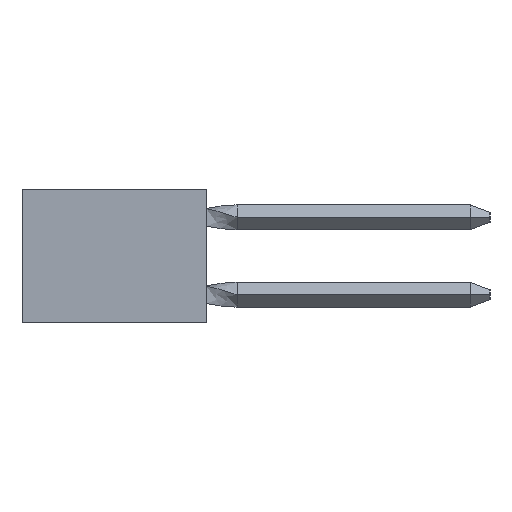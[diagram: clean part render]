
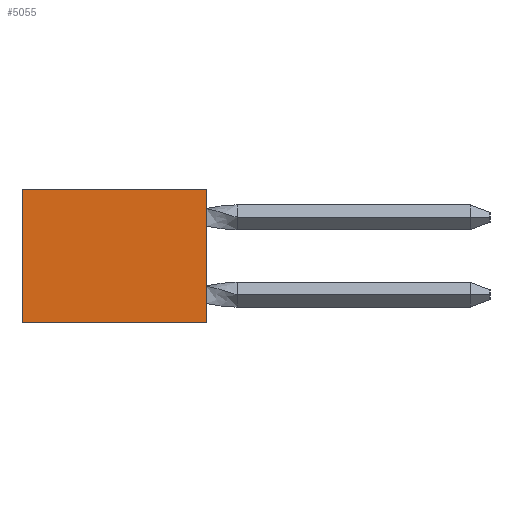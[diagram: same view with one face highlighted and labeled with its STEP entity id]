
A CAD part, left-side view. The second image highlights one B-rep face of the part: STEP entity #5055.
In plain terms, the highlighted planar face has unit normal (-1, 0, 0).
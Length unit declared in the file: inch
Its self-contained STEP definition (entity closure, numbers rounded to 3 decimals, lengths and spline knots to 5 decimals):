
#191 = VERTEX_POINT ( 'NONE', #24496 ) ;
#1643 = VECTOR ( 'NONE', #4269, 39.37008 ) ;
#1875 = LINE ( 'NONE', #1913, #13881 ) ;
#1913 = CARTESIAN_POINT ( 'NONE',  ( 0.298, 0., -0.343 ) ) ;
#3463 = DIRECTION ( 'NONE',  ( 0., 0., -1. ) ) ;
#4269 = DIRECTION ( 'NONE',  ( 0., 1., 0. ) ) ;
#5055 = ADVANCED_FACE ( 'NONE', ( #32895 ), #6270, .F. ) ;
#5742 = DIRECTION ( 'NONE',  ( 0., 0., -1. ) ) ;
#6270 = PLANE ( 'NONE',  #29863 ) ;
#7224 = CARTESIAN_POINT ( 'NONE',  ( 0.298, -0.027, 0. ) ) ;
#9084 = ORIENTED_EDGE ( 'NONE', *, *, #33490, .F. ) ;
#12258 = EDGE_LOOP ( 'NONE', ( #24165, #40208, #29659, #9084 ) ) ;
#12796 = LINE ( 'NONE', #31909, #51866 ) ;
#13763 = CARTESIAN_POINT ( 'NONE',  ( 0.298, 0.473, -0.343 ) ) ;
#13881 = VECTOR ( 'NONE', #32530, 39.37008 ) ;
#23214 = CARTESIAN_POINT ( 'NONE',  ( 0.298, 0.473, 0. ) ) ;
#24165 = ORIENTED_EDGE ( 'NONE', *, *, #41293, .T. ) ;
#24496 = CARTESIAN_POINT ( 'NONE',  ( 0.298, 0., -0.343 ) ) ;
#29659 = ORIENTED_EDGE ( 'NONE', *, *, #47153, .T. ) ;
#29863 = AXIS2_PLACEMENT_3D ( 'NONE', #54044, #36560, #3463 ) ;
#30447 = VERTEX_POINT ( 'NONE', #23214 ) ;
#31909 = CARTESIAN_POINT ( 'NONE',  ( 0.298, 0.473, 0. ) ) ;
#32014 = EDGE_CURVE ( 'NONE', #36370, #30447, #43511, .T. ) ;
#32530 = DIRECTION ( 'NONE',  ( 0., 0., 1. ) ) ;
#32895 = FACE_OUTER_BOUND ( 'NONE', #12258, .T. ) ;
#33490 = EDGE_CURVE ( 'NONE', #191, #38384, #52747, .T. ) ;
#36370 = VERTEX_POINT ( 'NONE', #36908 ) ;
#36560 = DIRECTION ( 'NONE',  ( 1., 0., 0. ) ) ;
#36908 = CARTESIAN_POINT ( 'NONE',  ( 0.298, 0., 0. ) ) ;
#38384 = VERTEX_POINT ( 'NONE', #13763 ) ;
#40208 = ORIENTED_EDGE ( 'NONE', *, *, #32014, .T. ) ;
#41293 = EDGE_CURVE ( 'NONE', #191, #36370, #1875, .T. ) ;
#43511 = LINE ( 'NONE', #7224, #44866 ) ;
#44866 = VECTOR ( 'NONE', #54224, 39.37008 ) ;
#47153 = EDGE_CURVE ( 'NONE', #30447, #38384, #12796, .T. ) ;
#51866 = VECTOR ( 'NONE', #5742, 39.37008 ) ;
#52747 = LINE ( 'NONE', #55390, #1643 ) ;
#54044 = CARTESIAN_POINT ( 'NONE',  ( 0.298, -0.027, 0. ) ) ;
#54224 = DIRECTION ( 'NONE',  ( 0., 1., 0. ) ) ;
#55390 = CARTESIAN_POINT ( 'NONE',  ( 0.298, 0.473, -0.343 ) ) ;
